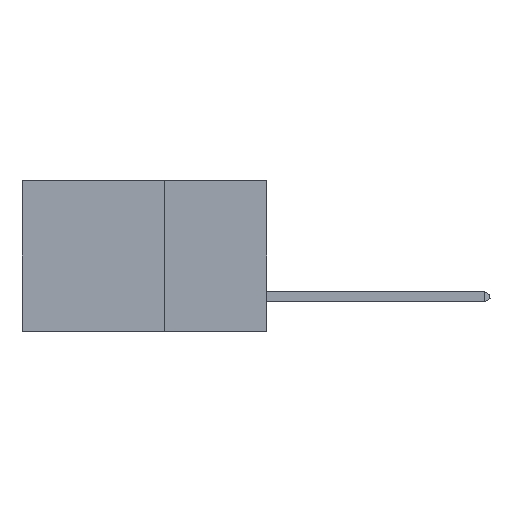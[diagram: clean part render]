
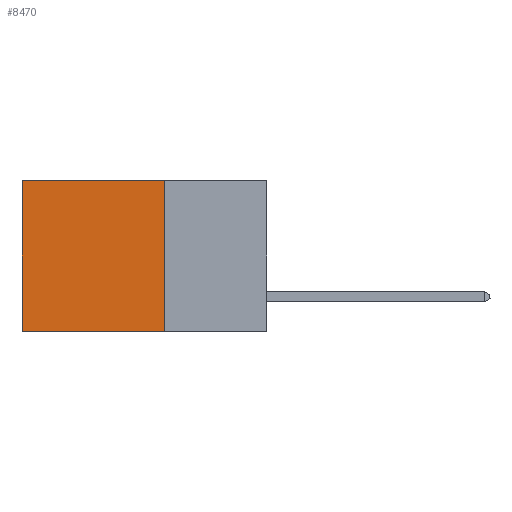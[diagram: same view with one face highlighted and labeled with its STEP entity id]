
A CAD part, left-side view. The second image highlights one B-rep face of the part: STEP entity #8470.
In plain terms, the highlighted planar face has unit normal (-1, 0, 0).
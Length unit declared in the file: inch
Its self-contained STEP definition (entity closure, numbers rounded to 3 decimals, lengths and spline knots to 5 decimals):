
#326 = EDGE_CURVE ( 'NONE', #3484, #1887, #40610, .T. ) ;
#1512 = ORIENTED_EDGE ( 'NONE', *, *, #43845, .F. ) ;
#1887 = VERTEX_POINT ( 'NONE', #9668 ) ;
#3484 = VERTEX_POINT ( 'NONE', #8035 ) ;
#4605 = VERTEX_POINT ( 'NONE', #9743 ) ;
#5785 = EDGE_CURVE ( 'NONE', #4605, #1887, #40870, .T. ) ;
#8035 = CARTESIAN_POINT ( 'NONE',  ( 0.2875, 0.25, -0.37 ) ) ;
#8470 = ADVANCED_FACE ( 'NONE', ( #9912 ), #18252, .F. ) ;
#9668 = CARTESIAN_POINT ( 'NONE',  ( 0.2875, 0.6, -0.37 ) ) ;
#9743 = CARTESIAN_POINT ( 'NONE',  ( 0.2875, 0.6, 0. ) ) ;
#9912 = FACE_OUTER_BOUND ( 'NONE', #14797, .T. ) ;
#11562 = CARTESIAN_POINT ( 'NONE',  ( 0.2875, 0.25, 0. ) ) ;
#14797 = EDGE_LOOP ( 'NONE', ( #25628, #43631, #1512, #41144 ) ) ;
#18252 = PLANE ( 'NONE',  #44560 ) ;
#18404 = DIRECTION ( 'NONE',  ( 0., 0., -1. ) ) ;
#25628 = ORIENTED_EDGE ( 'NONE', *, *, #5785, .T. ) ;
#27642 = LINE ( 'NONE', #29372, #33121 ) ;
#28519 = DIRECTION ( 'NONE',  ( 1., 0., 0. ) ) ;
#29046 = CARTESIAN_POINT ( 'NONE',  ( 0.2875, 0.25, 0. ) ) ;
#29372 = CARTESIAN_POINT ( 'NONE',  ( 0.2875, 0.25, 0. ) ) ;
#30252 = LINE ( 'NONE', #30447, #37269 ) ;
#30285 = VECTOR ( 'NONE', #31046, 39.37008 ) ;
#30447 = CARTESIAN_POINT ( 'NONE',  ( 0.2875, 0.25, 0. ) ) ;
#31046 = DIRECTION ( 'NONE',  ( 0., 1., 0. ) ) ;
#31625 = VECTOR ( 'NONE', #31771, 39.37008 ) ;
#31771 = DIRECTION ( 'NONE',  ( 0., 0., -1. ) ) ;
#33121 = VECTOR ( 'NONE', #36348, 39.37008 ) ;
#35080 = VERTEX_POINT ( 'NONE', #29046 ) ;
#36348 = DIRECTION ( 'NONE',  ( 0., 1., 0. ) ) ;
#37269 = VECTOR ( 'NONE', #43953, 39.37008 ) ;
#40610 = LINE ( 'NONE', #41356, #30285 ) ;
#40870 = LINE ( 'NONE', #42084, #31625 ) ;
#41144 = ORIENTED_EDGE ( 'NONE', *, *, #42226, .T. ) ;
#41356 = CARTESIAN_POINT ( 'NONE',  ( 0.2875, 0.25, -0.37 ) ) ;
#42084 = CARTESIAN_POINT ( 'NONE',  ( 0.2875, 0.6, 0. ) ) ;
#42226 = EDGE_CURVE ( 'NONE', #35080, #4605, #27642, .T. ) ;
#43631 = ORIENTED_EDGE ( 'NONE', *, *, #326, .F. ) ;
#43845 = EDGE_CURVE ( 'NONE', #35080, #3484, #30252, .T. ) ;
#43953 = DIRECTION ( 'NONE',  ( 0., 0., -1. ) ) ;
#44560 = AXIS2_PLACEMENT_3D ( 'NONE', #11562, #28519, #18404 ) ;
